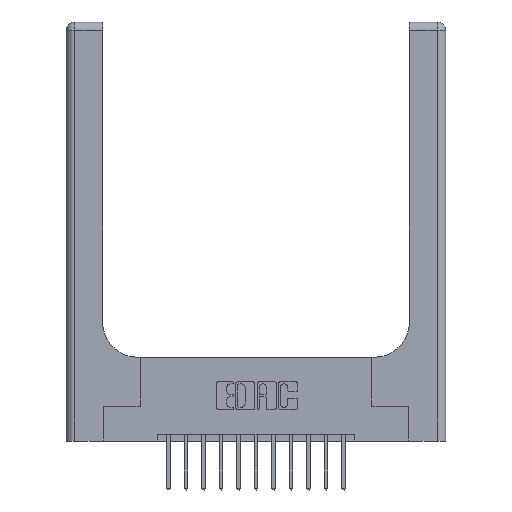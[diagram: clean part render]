
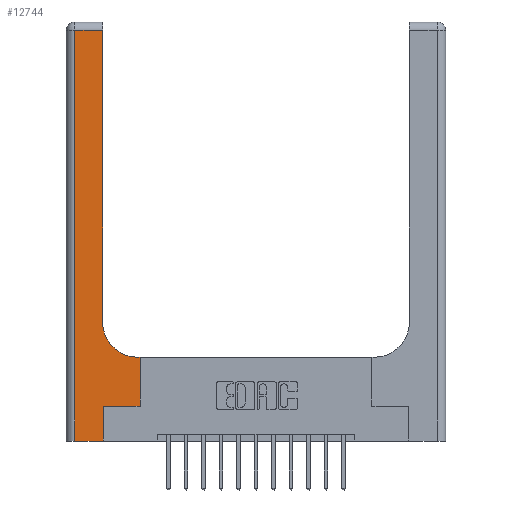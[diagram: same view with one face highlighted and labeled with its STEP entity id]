
A CAD part, top view. The second image highlights one B-rep face of the part: STEP entity #12744.
In plain terms, the highlighted planar face has unit normal (0, 0, 1).
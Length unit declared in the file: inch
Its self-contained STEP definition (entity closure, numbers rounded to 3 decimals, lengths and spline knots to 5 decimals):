
#154 = ORIENTED_EDGE ( 'NONE', *, *, #4741, .T. ) ;
#227 = ORIENTED_EDGE ( 'NONE', *, *, #12637, .T. ) ;
#339 = EDGE_LOOP ( 'NONE', ( #8103, #12091, #227, #154, #11245, #11223, #14626, #3202, #12552 ) ) ;
#377 = DIRECTION ( 'NONE',  ( -1., 0., 0. ) ) ;
#533 = CARTESIAN_POINT ( 'NONE',  ( 0.06, 3., 0.37 ) ) ;
#614 = VERTEX_POINT ( 'NONE', #2446 ) ;
#630 = LINE ( 'NONE', #13469, #677 ) ;
#677 = VECTOR ( 'NONE', #377, 39.37008 ) ;
#1058 = DIRECTION ( 'NONE',  ( -1., 0., 0. ) ) ;
#1197 = DIRECTION ( 'NONE',  ( 1., 0., 0. ) ) ;
#1447 = DIRECTION ( 'NONE',  ( 0., 1., 0. ) ) ;
#1711 = VERTEX_POINT ( 'NONE', #11890 ) ;
#1825 = AXIS2_PLACEMENT_3D ( 'NONE', #9940, #7552, #1058 ) ;
#2446 = CARTESIAN_POINT ( 'NONE',  ( 0.528, 0.25, 0.37 ) ) ;
#2510 = VECTOR ( 'NONE', #1197, 39.37008 ) ;
#2571 = CARTESIAN_POINT ( 'NONE',  ( 0.528, 0.6, 0.37 ) ) ;
#2573 = LINE ( 'NONE', #7687, #2510 ) ;
#2627 = DIRECTION ( 'NONE',  ( -1., 0., 0. ) ) ;
#3182 = DIRECTION ( 'NONE',  ( 1., 0., 0. ) ) ;
#3202 = ORIENTED_EDGE ( 'NONE', *, *, #6018, .T. ) ;
#3362 = EDGE_CURVE ( 'NONE', #1711, #7291, #9108, .T. ) ;
#3420 = DIRECTION ( 'NONE',  ( 0., 0., -1. ) ) ;
#3537 = CIRCLE ( 'NONE', #5715, 0.25 ) ;
#3734 = PLANE ( 'NONE',  #1825 ) ;
#3874 = CARTESIAN_POINT ( 'NONE',  ( 0.26, 0.85, 0.37 ) ) ;
#3932 = EDGE_CURVE ( 'NONE', #614, #7468, #10311, .T. ) ;
#4088 = EDGE_CURVE ( 'NONE', #8627, #1711, #12342, .T. ) ;
#4406 = DIRECTION ( 'NONE',  ( 0., 1., 0. ) ) ;
#4688 = VECTOR ( 'NONE', #13291, 39.37008 ) ;
#4741 = EDGE_CURVE ( 'NONE', #7979, #10911, #2573, .T. ) ;
#4936 = VECTOR ( 'NONE', #4406, 39.37008 ) ;
#5068 = VECTOR ( 'NONE', #1447, 39.37008 ) ;
#5444 = CARTESIAN_POINT ( 'NONE',  ( 0.265, 0., 0.37 ) ) ;
#5715 = AXIS2_PLACEMENT_3D ( 'NONE', #11410, #3420, #8675 ) ;
#6018 = EDGE_CURVE ( 'NONE', #7468, #9444, #630, .T. ) ;
#7291 = VERTEX_POINT ( 'NONE', #11006 ) ;
#7293 = FACE_OUTER_BOUND ( 'NONE', #339, .T. ) ;
#7468 = VERTEX_POINT ( 'NONE', #2571 ) ;
#7552 = DIRECTION ( 'NONE',  ( 0., 0., -1. ) ) ;
#7619 = CARTESIAN_POINT ( 'NONE',  ( 0.06, 0., 0.37 ) ) ;
#7687 = CARTESIAN_POINT ( 'NONE',  ( 0., 0., 0.37 ) ) ;
#7761 = CARTESIAN_POINT ( 'NONE',  ( 0.528, 0.25, 0.37 ) ) ;
#7889 = VECTOR ( 'NONE', #13701, 39.37008 ) ;
#7979 = VERTEX_POINT ( 'NONE', #7619 ) ;
#8103 = ORIENTED_EDGE ( 'NONE', *, *, #4088, .T. ) ;
#8159 = VECTOR ( 'NONE', #2627, 39.37008 ) ;
#8360 = LINE ( 'NONE', #11013, #16098 ) ;
#8627 = VERTEX_POINT ( 'NONE', #3874 ) ;
#8675 = DIRECTION ( 'NONE',  ( 1., 0., 0. ) ) ;
#8810 = EDGE_CURVE ( 'NONE', #10911, #16799, #12103, .T. ) ;
#8952 = EDGE_CURVE ( 'NONE', #9444, #8627, #3537, .T. ) ;
#9108 = LINE ( 'NONE', #9189, #8159 ) ;
#9189 = CARTESIAN_POINT ( 'NONE',  ( 0., 2.94, 0.37 ) ) ;
#9444 = VERTEX_POINT ( 'NONE', #13714 ) ;
#9711 = CARTESIAN_POINT ( 'NONE',  ( 0.26, 3., 0.37 ) ) ;
#9940 = CARTESIAN_POINT ( 'NONE',  ( 0., 3., 0.37 ) ) ;
#10311 = LINE ( 'NONE', #7761, #5068 ) ;
#10790 = LINE ( 'NONE', #533, #7889 ) ;
#10857 = CARTESIAN_POINT ( 'NONE',  ( 0.265, 0.25, 0.37 ) ) ;
#10911 = VERTEX_POINT ( 'NONE', #11749 ) ;
#11006 = CARTESIAN_POINT ( 'NONE',  ( 0.06, 2.94, 0.37 ) ) ;
#11013 = CARTESIAN_POINT ( 'NONE',  ( 0.265, 0.25, 0.37 ) ) ;
#11223 = ORIENTED_EDGE ( 'NONE', *, *, #13024, .T. ) ;
#11245 = ORIENTED_EDGE ( 'NONE', *, *, #8810, .T. ) ;
#11410 = CARTESIAN_POINT ( 'NONE',  ( 0.51, 0.85, 0.37 ) ) ;
#11749 = CARTESIAN_POINT ( 'NONE',  ( 0.265, 0., 0.37 ) ) ;
#11890 = CARTESIAN_POINT ( 'NONE',  ( 0.26, 2.94, 0.37 ) ) ;
#12091 = ORIENTED_EDGE ( 'NONE', *, *, #3362, .T. ) ;
#12103 = LINE ( 'NONE', #5444, #4936 ) ;
#12342 = LINE ( 'NONE', #9711, #4688 ) ;
#12552 = ORIENTED_EDGE ( 'NONE', *, *, #8952, .T. ) ;
#12637 = EDGE_CURVE ( 'NONE', #7291, #7979, #10790, .T. ) ;
#12744 = ADVANCED_FACE ( 'NONE', ( #7293 ), #3734, .F. ) ;
#13024 = EDGE_CURVE ( 'NONE', #16799, #614, #8360, .T. ) ;
#13291 = DIRECTION ( 'NONE',  ( 0., 1., 0. ) ) ;
#13469 = CARTESIAN_POINT ( 'NONE',  ( 0.26, 0.6, 0.37 ) ) ;
#13701 = DIRECTION ( 'NONE',  ( 0., -1., 0. ) ) ;
#13714 = CARTESIAN_POINT ( 'NONE',  ( 0.51, 0.6, 0.37 ) ) ;
#14626 = ORIENTED_EDGE ( 'NONE', *, *, #3932, .T. ) ;
#16098 = VECTOR ( 'NONE', #3182, 39.37008 ) ;
#16799 = VERTEX_POINT ( 'NONE', #10857 ) ;
